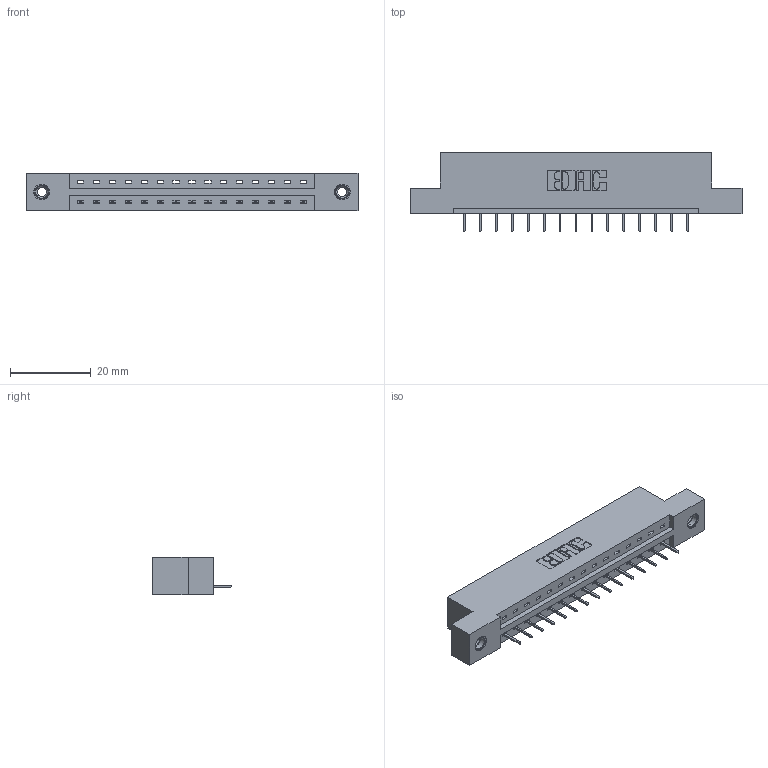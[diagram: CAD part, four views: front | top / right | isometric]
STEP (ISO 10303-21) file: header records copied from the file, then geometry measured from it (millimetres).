
FILE_DESCRIPTION (( 'STEP AP203' ), '1' );
FILE_NAME ('387-015-524-108.STEP', '2018-09-11T07:28:38', ( '' ), ( '' ), 'SwSTEP 2.0', 'SolidWorks 2016', '' );
FILE_SCHEMA (( 'CONFIG_CONTROL_DESIGN' ));
Length unit declared in the file: inch
Products named in the file (4): 337 Part_Flush Mounting Lugs - 0.156 Dia-TI; 345-292-001_345-293-124; 345-250-001_345-250-003-102; 387-015-524-108
Assembly tree (18 placements, depth 2):
  387-015-524-108
    337 Part_Flush Mounting Lugs - 0.156 Dia-TI
    345-292-001_345-293-124  x15
    345-250-001_345-250-003-102  x2
Bounding box: 82.45 x 19.69 x 9.4 mm (x, y, z)
Volume: 8165.5 mm3; surface area: 8109.3 mm2
Topology: 18 solids, 18 shells, 1164 faces, 3327 edges, 2150 vertices
Faces by surface type: plane 882, cylinder 266, cone 12, torus 4
Entity records: 15902 total; most frequent: CARTESIAN_POINT 2746, ORIENTED_EDGE 2690, DIRECTION 2401, EDGE_CURVE 1345, LINE 1201, VECTOR 1201, VERTEX_POINT 888, AXIS2_PLACEMENT_3D 600
